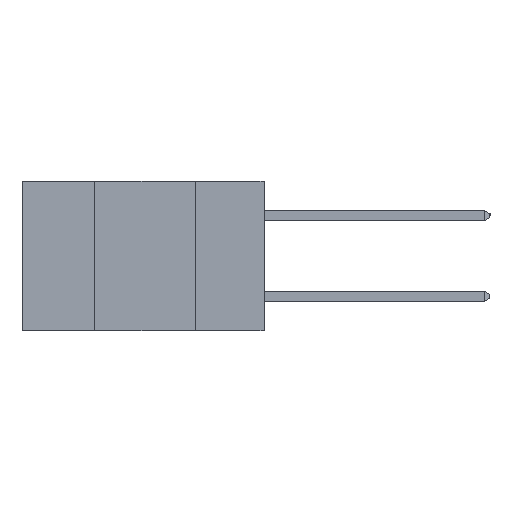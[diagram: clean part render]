
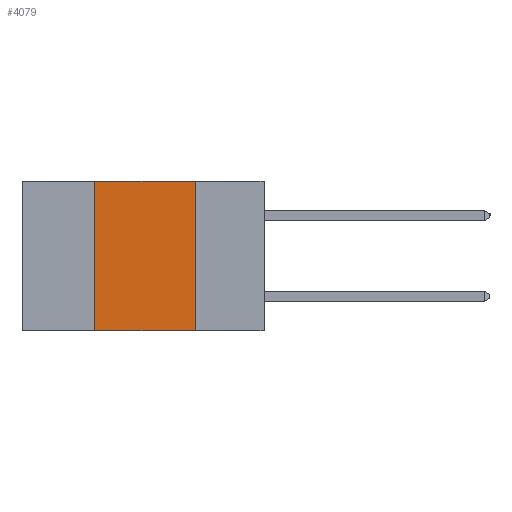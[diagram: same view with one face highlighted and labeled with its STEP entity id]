
A CAD part, left-side view. The second image highlights one B-rep face of the part: STEP entity #4079.
In plain terms, the highlighted planar face has unit normal (-1, 0, 0).
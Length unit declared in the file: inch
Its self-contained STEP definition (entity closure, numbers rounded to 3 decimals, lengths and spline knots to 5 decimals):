
#505 = EDGE_CURVE ( 'NONE', #19130, #8259, #18169, .T. ) ;
#1775 = CARTESIAN_POINT ( 'NONE',  ( 0., 0.6, 0. ) ) ;
#1879 = EDGE_CURVE ( 'NONE', #5574, #20583, #10990, .T. ) ;
#1987 = ORIENTED_EDGE ( 'NONE', *, *, #9486, .F. ) ;
#2549 = ORIENTED_EDGE ( 'NONE', *, *, #22165, .F. ) ;
#2655 = CARTESIAN_POINT ( 'NONE',  ( 0., 0.17, -0.37 ) ) ;
#3391 = DIRECTION ( 'NONE',  ( 0., 0., -1. ) ) ;
#3631 = AXIS2_PLACEMENT_3D ( 'NONE', #7585, #9738, #16691 ) ;
#3979 = PLANE ( 'NONE',  #3631 ) ;
#4079 = ADVANCED_FACE ( 'NONE', ( #14986 ), #3979, .F. ) ;
#5574 = VERTEX_POINT ( 'NONE', #17649 ) ;
#6348 = CARTESIAN_POINT ( 'NONE',  ( 0., 0.42, 0. ) ) ;
#6760 = LINE ( 'NONE', #14054, #21302 ) ;
#6934 = EDGE_LOOP ( 'NONE', ( #1987, #12921, #2549, #9470 ) ) ;
#7585 = CARTESIAN_POINT ( 'NONE',  ( 0., 0.6, 0. ) ) ;
#8259 = VERTEX_POINT ( 'NONE', #11131 ) ;
#9470 = ORIENTED_EDGE ( 'NONE', *, *, #1879, .T. ) ;
#9486 = EDGE_CURVE ( 'NONE', #8259, #20583, #23011, .T. ) ;
#9704 = VECTOR ( 'NONE', #18401, 39.37008 ) ;
#9738 = DIRECTION ( 'NONE',  ( 1., 0., 0. ) ) ;
#10990 = LINE ( 'NONE', #18295, #9704 ) ;
#11131 = CARTESIAN_POINT ( 'NONE',  ( 0., 0.17, 0. ) ) ;
#12921 = ORIENTED_EDGE ( 'NONE', *, *, #505, .F. ) ;
#14054 = CARTESIAN_POINT ( 'NONE',  ( 0., 0.42, -0.37 ) ) ;
#14986 = FACE_OUTER_BOUND ( 'NONE', #6934, .T. ) ;
#16691 = DIRECTION ( 'NONE',  ( 0., 0., -1. ) ) ;
#17649 = CARTESIAN_POINT ( 'NONE',  ( 0., 0.42, -0.37 ) ) ;
#17821 = DIRECTION ( 'NONE',  ( 0., -1., 0. ) ) ;
#18009 = CARTESIAN_POINT ( 'NONE',  ( 0., 0.17, -0.37 ) ) ;
#18022 = DIRECTION ( 'NONE',  ( 0., 0., 1. ) ) ;
#18169 = LINE ( 'NONE', #1775, #19798 ) ;
#18295 = CARTESIAN_POINT ( 'NONE',  ( 0., 0.6, -0.37 ) ) ;
#18401 = DIRECTION ( 'NONE',  ( 0., -1., 0. ) ) ;
#19130 = VERTEX_POINT ( 'NONE', #6348 ) ;
#19220 = VECTOR ( 'NONE', #3391, 39.37008 ) ;
#19798 = VECTOR ( 'NONE', #17821, 39.37008 ) ;
#20583 = VERTEX_POINT ( 'NONE', #2655 ) ;
#21302 = VECTOR ( 'NONE', #18022, 39.37008 ) ;
#22165 = EDGE_CURVE ( 'NONE', #5574, #19130, #6760, .T. ) ;
#23011 = LINE ( 'NONE', #18009, #19220 ) ;
